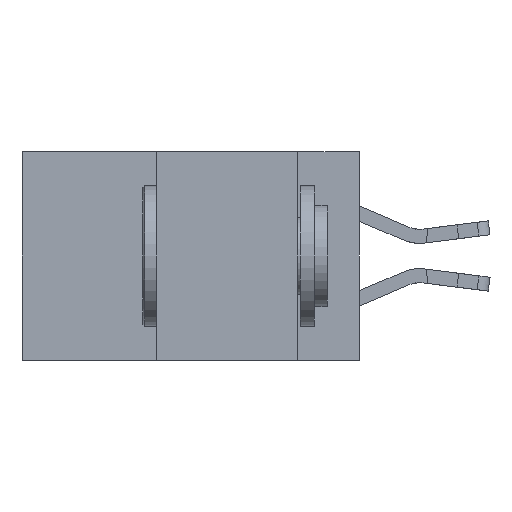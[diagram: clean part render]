
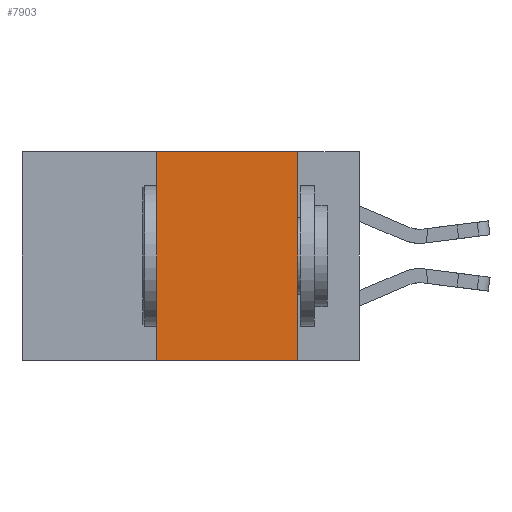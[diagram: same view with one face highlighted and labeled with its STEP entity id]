
A CAD part, left-side view. The second image highlights one B-rep face of the part: STEP entity #7903.
In plain terms, the highlighted planar face has unit normal (-1, 0, 0).
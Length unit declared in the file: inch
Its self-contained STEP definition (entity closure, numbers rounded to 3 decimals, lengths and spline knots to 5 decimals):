
#1229 = LINE ( 'NONE', #29291, #27456 ) ;
#4061 = DIRECTION ( 'NONE',  ( 1., 0., 0. ) ) ;
#5985 = VECTOR ( 'NONE', #18397, 39.37008 ) ;
#6281 = ORIENTED_EDGE ( 'NONE', *, *, #10851, .F. ) ;
#7903 = ADVANCED_FACE ( 'NONE', ( #21583 ), #31726, .F. ) ;
#8161 = CARTESIAN_POINT ( 'NONE',  ( 0., 0.36, 0. ) ) ;
#8305 = VECTOR ( 'NONE', #17551, 39.37008 ) ;
#8659 = LINE ( 'NONE', #20397, #21409 ) ;
#9155 = EDGE_CURVE ( 'NONE', #29262, #20737, #1229, .T. ) ;
#9726 = VERTEX_POINT ( 'NONE', #11218 ) ;
#10851 = EDGE_CURVE ( 'NONE', #9726, #29262, #31964, .T. ) ;
#11218 = CARTESIAN_POINT ( 'NONE',  ( 0., 0.36, -0.37 ) ) ;
#11344 = VERTEX_POINT ( 'NONE', #32616 ) ;
#14021 = ORIENTED_EDGE ( 'NONE', *, *, #19191, .T. ) ;
#15017 = CARTESIAN_POINT ( 'NONE',  ( 0., 0.11, 0. ) ) ;
#17551 = DIRECTION ( 'NONE',  ( 0., 0., -1. ) ) ;
#18397 = DIRECTION ( 'NONE',  ( 0., 0., 1. ) ) ;
#19191 = EDGE_CURVE ( 'NONE', #9726, #11344, #8659, .T. ) ;
#20397 = CARTESIAN_POINT ( 'NONE',  ( 0., 0.6, -0.37 ) ) ;
#20737 = VERTEX_POINT ( 'NONE', #26534 ) ;
#20984 = AXIS2_PLACEMENT_3D ( 'NONE', #29149, #4061, #21930 ) ;
#21409 = VECTOR ( 'NONE', #30308, 39.37008 ) ;
#21583 = FACE_OUTER_BOUND ( 'NONE', #30127, .T. ) ;
#21858 = LINE ( 'NONE', #15017, #8305 ) ;
#21930 = DIRECTION ( 'NONE',  ( 0., 0., -1. ) ) ;
#22180 = CARTESIAN_POINT ( 'NONE',  ( 0., 0.36, 0. ) ) ;
#25726 = ORIENTED_EDGE ( 'NONE', *, *, #28692, .F. ) ;
#26534 = CARTESIAN_POINT ( 'NONE',  ( 0., 0.11, 0. ) ) ;
#27456 = VECTOR ( 'NONE', #31768, 39.37008 ) ;
#28692 = EDGE_CURVE ( 'NONE', #20737, #11344, #21858, .T. ) ;
#29149 = CARTESIAN_POINT ( 'NONE',  ( 0., 0.6, 0. ) ) ;
#29262 = VERTEX_POINT ( 'NONE', #22180 ) ;
#29291 = CARTESIAN_POINT ( 'NONE',  ( 0., 0.6, 0. ) ) ;
#30127 = EDGE_LOOP ( 'NONE', ( #25726, #32254, #6281, #14021 ) ) ;
#30308 = DIRECTION ( 'NONE',  ( 0., -1., 0. ) ) ;
#31726 = PLANE ( 'NONE',  #20984 ) ;
#31768 = DIRECTION ( 'NONE',  ( 0., -1., 0. ) ) ;
#31964 = LINE ( 'NONE', #8161, #5985 ) ;
#32254 = ORIENTED_EDGE ( 'NONE', *, *, #9155, .F. ) ;
#32616 = CARTESIAN_POINT ( 'NONE',  ( 0., 0.11, -0.37 ) ) ;
